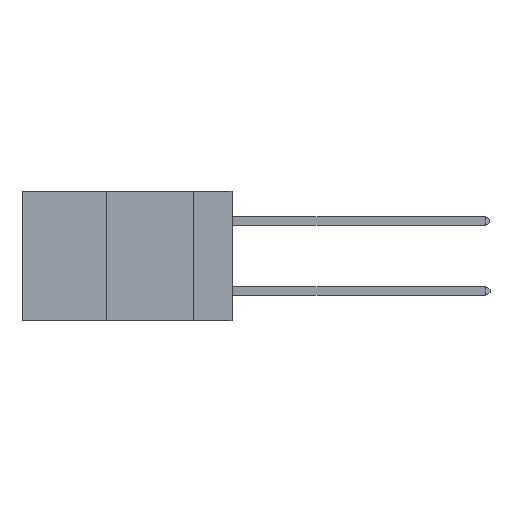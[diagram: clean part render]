
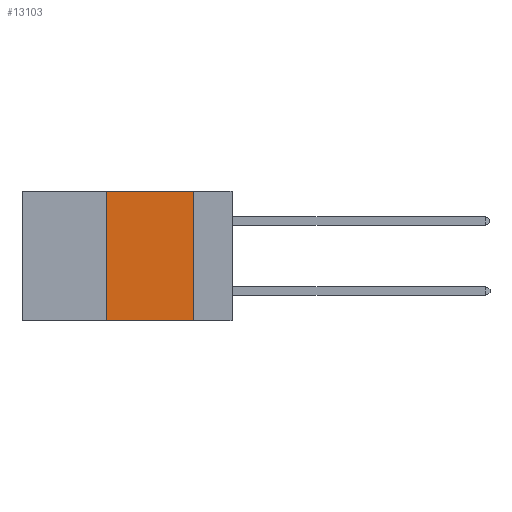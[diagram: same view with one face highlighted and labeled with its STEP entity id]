
A CAD part, left-side view. The second image highlights one B-rep face of the part: STEP entity #13103.
In plain terms, the highlighted planar face has unit normal (-1, 0, 0).
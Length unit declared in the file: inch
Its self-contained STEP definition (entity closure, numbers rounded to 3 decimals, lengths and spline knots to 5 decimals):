
#1251 = CARTESIAN_POINT ( 'NONE',  ( 0., 0.11, -0.37 ) ) ;
#1393 = DIRECTION ( 'NONE',  ( 1., 0., 0. ) ) ;
#2562 = VECTOR ( 'NONE', #4389, 39.37008 ) ;
#2589 = CARTESIAN_POINT ( 'NONE',  ( 0., 0.36, -0.37 ) ) ;
#2664 = CARTESIAN_POINT ( 'NONE',  ( 0., 0.36, 0. ) ) ;
#2789 = LINE ( 'NONE', #9491, #4987 ) ;
#2886 = LINE ( 'NONE', #2664, #2562 ) ;
#3286 = ORIENTED_EDGE ( 'NONE', *, *, #5006, .F. ) ;
#3520 = CARTESIAN_POINT ( 'NONE',  ( 0., 0.11, 0. ) ) ;
#3599 = VECTOR ( 'NONE', #12813, 39.37008 ) ;
#3925 = VERTEX_POINT ( 'NONE', #6142 ) ;
#4389 = DIRECTION ( 'NONE',  ( 0., 0., 1. ) ) ;
#4467 = EDGE_LOOP ( 'NONE', ( #7909, #11151, #3286, #9774 ) ) ;
#4581 = AXIS2_PLACEMENT_3D ( 'NONE', #5749, #1393, #8816 ) ;
#4949 = EDGE_CURVE ( 'NONE', #11026, #7500, #9101, .T. ) ;
#4987 = VECTOR ( 'NONE', #10540, 39.37008 ) ;
#5006 = EDGE_CURVE ( 'NONE', #11026, #3925, #2886, .T. ) ;
#5066 = EDGE_CURVE ( 'NONE', #10110, #7500, #12807, .T. ) ;
#5749 = CARTESIAN_POINT ( 'NONE',  ( 0., 0.6, 0. ) ) ;
#6142 = CARTESIAN_POINT ( 'NONE',  ( 0., 0.36, 0. ) ) ;
#6631 = DIRECTION ( 'NONE',  ( 0., 0., -1. ) ) ;
#6818 = PLANE ( 'NONE',  #4581 ) ;
#6886 = CARTESIAN_POINT ( 'NONE',  ( 0., 0.6, -0.37 ) ) ;
#7500 = VERTEX_POINT ( 'NONE', #1251 ) ;
#7683 = FACE_OUTER_BOUND ( 'NONE', #4467, .T. ) ;
#7909 = ORIENTED_EDGE ( 'NONE', *, *, #5066, .F. ) ;
#8300 = EDGE_CURVE ( 'NONE', #3925, #10110, #2789, .T. ) ;
#8816 = DIRECTION ( 'NONE',  ( 0., 0., -1. ) ) ;
#9101 = LINE ( 'NONE', #6886, #3599 ) ;
#9491 = CARTESIAN_POINT ( 'NONE',  ( 0., 0.6, 0. ) ) ;
#9774 = ORIENTED_EDGE ( 'NONE', *, *, #4949, .T. ) ;
#10110 = VERTEX_POINT ( 'NONE', #12290 ) ;
#10540 = DIRECTION ( 'NONE',  ( 0., -1., 0. ) ) ;
#11026 = VERTEX_POINT ( 'NONE', #2589 ) ;
#11151 = ORIENTED_EDGE ( 'NONE', *, *, #8300, .F. ) ;
#12290 = CARTESIAN_POINT ( 'NONE',  ( 0., 0.11, 0. ) ) ;
#12487 = VECTOR ( 'NONE', #6631, 39.37008 ) ;
#12807 = LINE ( 'NONE', #3520, #12487 ) ;
#12813 = DIRECTION ( 'NONE',  ( 0., -1., 0. ) ) ;
#13103 = ADVANCED_FACE ( 'NONE', ( #7683 ), #6818, .F. ) ;
